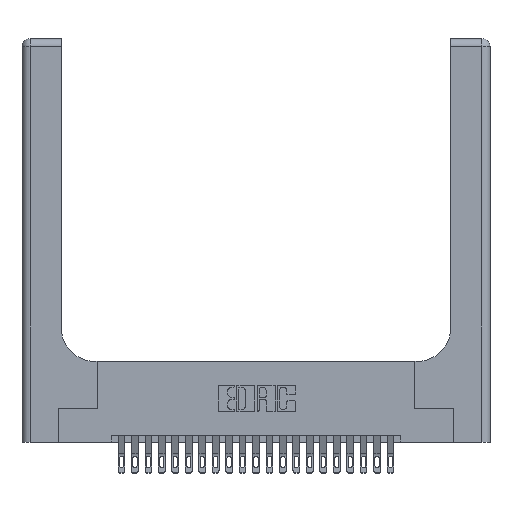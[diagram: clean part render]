
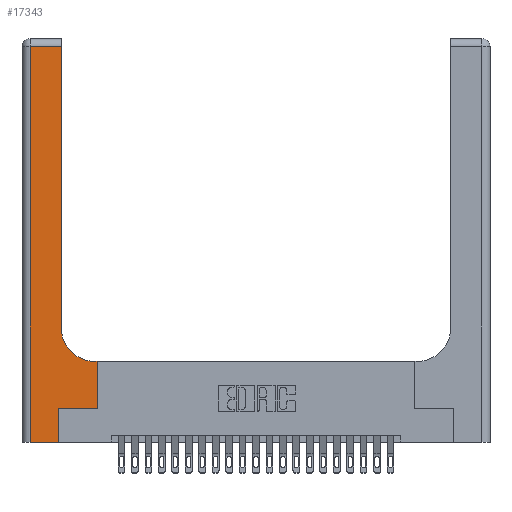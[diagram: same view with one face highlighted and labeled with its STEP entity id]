
A CAD part, top view. The second image highlights one B-rep face of the part: STEP entity #17343.
In plain terms, the highlighted planar face has unit normal (0, 0, 1).
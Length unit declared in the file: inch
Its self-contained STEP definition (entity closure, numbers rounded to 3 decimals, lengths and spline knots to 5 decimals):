
#155 = ORIENTED_EDGE ( 'NONE', *, *, #22459, .T. ) ;
#887 = DIRECTION ( 'NONE',  ( -1., 0., 0. ) ) ;
#1142 = ORIENTED_EDGE ( 'NONE', *, *, #12197, .T. ) ;
#1601 = LINE ( 'NONE', #12629, #12033 ) ;
#1627 = VERTEX_POINT ( 'NONE', #13316 ) ;
#1890 = DIRECTION ( 'NONE',  ( 1., 0., 0. ) ) ;
#1907 = CARTESIAN_POINT ( 'NONE',  ( 0.06, 3., 0.37 ) ) ;
#2482 = VERTEX_POINT ( 'NONE', #11531 ) ;
#2964 = DIRECTION ( 'NONE',  ( 1., 0., 0. ) ) ;
#3224 = EDGE_LOOP ( 'NONE', ( #8944, #15735, #10249, #22023, #17042, #24355, #155, #1142, #20677 ) ) ;
#3502 = LINE ( 'NONE', #24157, #17538 ) ;
#4299 = CARTESIAN_POINT ( 'NONE',  ( 0.269, 0.25, 0.37 ) ) ;
#4411 = PLANE ( 'NONE',  #19207 ) ;
#4772 = LINE ( 'NONE', #1907, #13759 ) ;
#4810 = VECTOR ( 'NONE', #11613, 39.37008 ) ;
#5018 = CARTESIAN_POINT ( 'NONE',  ( 0.2915, 2.94, 0.37 ) ) ;
#6522 = CARTESIAN_POINT ( 'NONE',  ( 0.5415, 0.85, 0.37 ) ) ;
#7901 = VERTEX_POINT ( 'NONE', #11487 ) ;
#7968 = EDGE_CURVE ( 'NONE', #23196, #9715, #23617, .T. ) ;
#7990 = VECTOR ( 'NONE', #2964, 39.37008 ) ;
#8334 = DIRECTION ( 'NONE',  ( -1., 0., 0. ) ) ;
#8456 = DIRECTION ( 'NONE',  ( 1., 0., 0. ) ) ;
#8873 = CIRCLE ( 'NONE', #20344, 0.25 ) ;
#8944 = ORIENTED_EDGE ( 'NONE', *, *, #22846, .T. ) ;
#9174 = VECTOR ( 'NONE', #23116, 39.37008 ) ;
#9207 = DIRECTION ( 'NONE',  ( 0., 1., 0. ) ) ;
#9212 = VERTEX_POINT ( 'NONE', #5018 ) ;
#9715 = VERTEX_POINT ( 'NONE', #14024 ) ;
#10054 = VECTOR ( 'NONE', #21884, 39.37008 ) ;
#10227 = EDGE_CURVE ( 'NONE', #14525, #2482, #8873, .T. ) ;
#10249 = ORIENTED_EDGE ( 'NONE', *, *, #13042, .T. ) ;
#10639 = LINE ( 'NONE', #19987, #10054 ) ;
#11487 = CARTESIAN_POINT ( 'NONE',  ( 0.269, 0., 0.37 ) ) ;
#11531 = CARTESIAN_POINT ( 'NONE',  ( 0.2915, 0.85, 0.37 ) ) ;
#11613 = DIRECTION ( 'NONE',  ( 0., 1., 0. ) ) ;
#11655 = CARTESIAN_POINT ( 'NONE',  ( 0.269, 0.25, 0.37 ) ) ;
#12033 = VECTOR ( 'NONE', #887, 39.37008 ) ;
#12197 = EDGE_CURVE ( 'NONE', #17038, #14525, #1601, .T. ) ;
#12629 = CARTESIAN_POINT ( 'NONE',  ( 0.2915, 0.6, 0.37 ) ) ;
#12920 = CARTESIAN_POINT ( 'NONE',  ( 0.5415, 0.6, 0.37 ) ) ;
#13042 = EDGE_CURVE ( 'NONE', #13897, #1627, #4772, .T. ) ;
#13316 = CARTESIAN_POINT ( 'NONE',  ( 0.06, 0., 0.37 ) ) ;
#13612 = LINE ( 'NONE', #22004, #7990 ) ;
#13759 = VECTOR ( 'NONE', #17162, 39.37008 ) ;
#13897 = VERTEX_POINT ( 'NONE', #23694 ) ;
#14024 = CARTESIAN_POINT ( 'NONE',  ( 0.5585, 0.25, 0.37 ) ) ;
#14525 = VERTEX_POINT ( 'NONE', #12920 ) ;
#14769 = LINE ( 'NONE', #19359, #9174 ) ;
#15031 = CARTESIAN_POINT ( 'NONE',  ( 0.5585, 0.6, 0.37 ) ) ;
#15735 = ORIENTED_EDGE ( 'NONE', *, *, #19627, .T. ) ;
#17038 = VERTEX_POINT ( 'NONE', #15031 ) ;
#17042 = ORIENTED_EDGE ( 'NONE', *, *, #19827, .T. ) ;
#17162 = DIRECTION ( 'NONE',  ( 0., -1., 0. ) ) ;
#17343 = ADVANCED_FACE ( 'NONE', ( #21050 ), #4411, .F. ) ;
#17538 = VECTOR ( 'NONE', #9207, 39.37008 ) ;
#17711 = CARTESIAN_POINT ( 'NONE',  ( 0., 3., 0.37 ) ) ;
#19207 = AXIS2_PLACEMENT_3D ( 'NONE', #17711, #19624, #8334 ) ;
#19223 = VECTOR ( 'NONE', #1890, 39.37008 ) ;
#19237 = EDGE_CURVE ( 'NONE', #1627, #7901, #13612, .T. ) ;
#19359 = CARTESIAN_POINT ( 'NONE',  ( 0., 2.94, 0.37 ) ) ;
#19624 = DIRECTION ( 'NONE',  ( 0., 0., -1. ) ) ;
#19627 = EDGE_CURVE ( 'NONE', #9212, #13897, #14769, .T. ) ;
#19721 = DIRECTION ( 'NONE',  ( 0., 0., -1. ) ) ;
#19827 = EDGE_CURVE ( 'NONE', #7901, #23196, #10639, .T. ) ;
#19950 = LINE ( 'NONE', #24716, #4810 ) ;
#19987 = CARTESIAN_POINT ( 'NONE',  ( 0.269, 0., 0.37 ) ) ;
#20344 = AXIS2_PLACEMENT_3D ( 'NONE', #6522, #19721, #8456 ) ;
#20677 = ORIENTED_EDGE ( 'NONE', *, *, #10227, .T. ) ;
#21050 = FACE_OUTER_BOUND ( 'NONE', #3224, .T. ) ;
#21884 = DIRECTION ( 'NONE',  ( 0., 1., 0. ) ) ;
#22004 = CARTESIAN_POINT ( 'NONE',  ( 0., 0., 0.37 ) ) ;
#22023 = ORIENTED_EDGE ( 'NONE', *, *, #19237, .T. ) ;
#22459 = EDGE_CURVE ( 'NONE', #9715, #17038, #19950, .T. ) ;
#22846 = EDGE_CURVE ( 'NONE', #2482, #9212, #3502, .T. ) ;
#23116 = DIRECTION ( 'NONE',  ( -1., 0., 0. ) ) ;
#23196 = VERTEX_POINT ( 'NONE', #4299 ) ;
#23617 = LINE ( 'NONE', #11655, #19223 ) ;
#23694 = CARTESIAN_POINT ( 'NONE',  ( 0.06, 2.94, 0.37 ) ) ;
#24157 = CARTESIAN_POINT ( 'NONE',  ( 0.2915, 3., 0.37 ) ) ;
#24355 = ORIENTED_EDGE ( 'NONE', *, *, #7968, .T. ) ;
#24716 = CARTESIAN_POINT ( 'NONE',  ( 0.5585, 0.25, 0.37 ) ) ;
